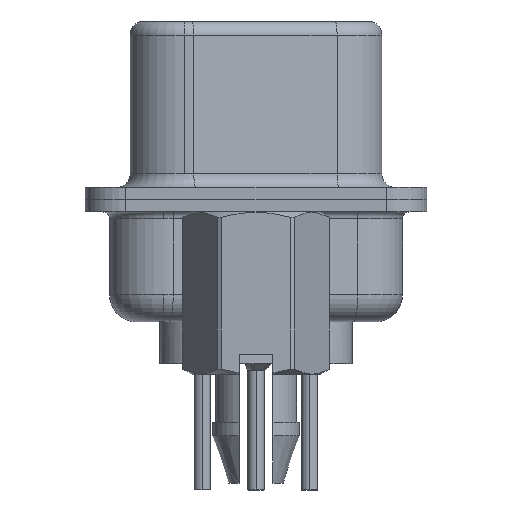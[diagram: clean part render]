
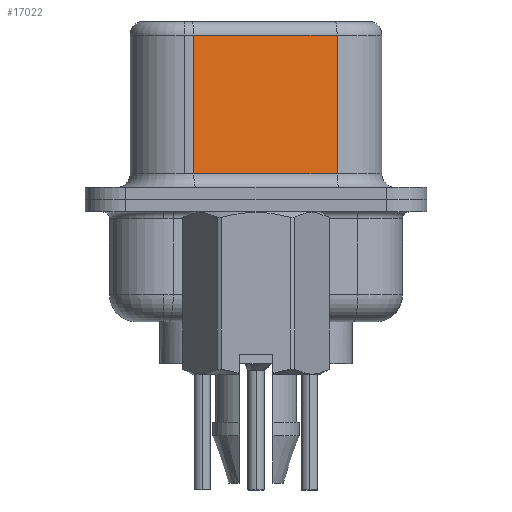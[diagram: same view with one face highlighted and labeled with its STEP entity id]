
A CAD part, left-side view. The second image highlights one B-rep face of the part: STEP entity #17022.
In plain terms, the highlighted planar face has unit normal (-0.985, -0.174, 0).
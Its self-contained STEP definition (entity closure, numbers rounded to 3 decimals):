
#531 = VERTEX_POINT ( 'NONE', #3291 ) ;
#955 = CARTESIAN_POINT ( 'NONE',  ( 4.546, -2.987, 6.57 ) ) ;
#1472 = DIRECTION ( 'NONE',  ( 0., 0., -1. ) ) ;
#3291 = CARTESIAN_POINT ( 'NONE',  ( 3.615, 2.293, 6.07 ) ) ;
#3327 = LINE ( 'NONE', #10913, #4945 ) ;
#4199 = PLANE ( 'NONE',  #5283 ) ;
#4353 = VERTEX_POINT ( 'NONE', #24416 ) ;
#4945 = VECTOR ( 'NONE', #1472, 1000. ) ;
#4980 = EDGE_CURVE ( 'NONE', #531, #17540, #3327, .T. ) ;
#5283 = AXIS2_PLACEMENT_3D ( 'NONE', #955, #17470, #17740 ) ;
#5540 = CARTESIAN_POINT ( 'NONE',  ( 4.546, -2.987, 0.95 ) ) ;
#6099 = ORIENTED_EDGE ( 'NONE', *, *, #4980, .T. ) ;
#6190 = EDGE_CURVE ( 'NONE', #17540, #15551, #6473, .T. ) ;
#6473 = LINE ( 'NONE', #11847, #16952 ) ;
#7139 = EDGE_CURVE ( 'NONE', #4353, #15551, #11645, .T. ) ;
#7808 = EDGE_CURVE ( 'NONE', #4353, #531, #12472, .T. ) ;
#7939 = VECTOR ( 'NONE', #18163, 1000. ) ;
#10605 = CARTESIAN_POINT ( 'NONE',  ( 4.546, -2.987, 6.07 ) ) ;
#10903 = EDGE_LOOP ( 'NONE', ( #24237, #12838, #6099, #17000 ) ) ;
#10913 = CARTESIAN_POINT ( 'NONE',  ( 3.615, 2.293, 6.57 ) ) ;
#11645 = LINE ( 'NONE', #17568, #21786 ) ;
#11847 = CARTESIAN_POINT ( 'NONE',  ( 4.546, -2.987, 0.95 ) ) ;
#12472 = LINE ( 'NONE', #10605, #7939 ) ;
#12838 = ORIENTED_EDGE ( 'NONE', *, *, #7808, .T. ) ;
#14054 = DIRECTION ( 'NONE',  ( 0.174, -0.985, 0. ) ) ;
#14197 = CARTESIAN_POINT ( 'NONE',  ( 3.615, 2.293, 0.95 ) ) ;
#15551 = VERTEX_POINT ( 'NONE', #5540 ) ;
#15705 = DIRECTION ( 'NONE',  ( 0., 0., -1. ) ) ;
#16952 = VECTOR ( 'NONE', #14054, 1000. ) ;
#17000 = ORIENTED_EDGE ( 'NONE', *, *, #6190, .T. ) ;
#17022 = ADVANCED_FACE ( 'NONE', ( #19600 ), #4199, .F. ) ;
#17470 = DIRECTION ( 'NONE',  ( 0.985, 0.174, 0. ) ) ;
#17540 = VERTEX_POINT ( 'NONE', #14197 ) ;
#17568 = CARTESIAN_POINT ( 'NONE',  ( 4.546, -2.987, 6.57 ) ) ;
#17740 = DIRECTION ( 'NONE',  ( -0.174, 0.985, 0. ) ) ;
#18163 = DIRECTION ( 'NONE',  ( -0.174, 0.985, 0. ) ) ;
#19600 = FACE_OUTER_BOUND ( 'NONE', #10903, .T. ) ;
#21786 = VECTOR ( 'NONE', #15705, 1000. ) ;
#24237 = ORIENTED_EDGE ( 'NONE', *, *, #7139, .F. ) ;
#24416 = CARTESIAN_POINT ( 'NONE',  ( 4.546, -2.987, 6.07 ) ) ;
